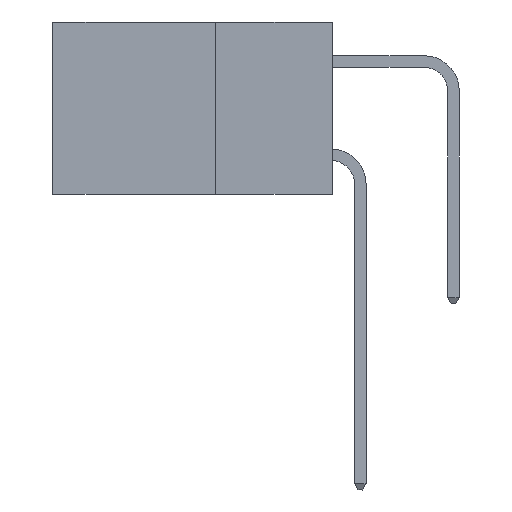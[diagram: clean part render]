
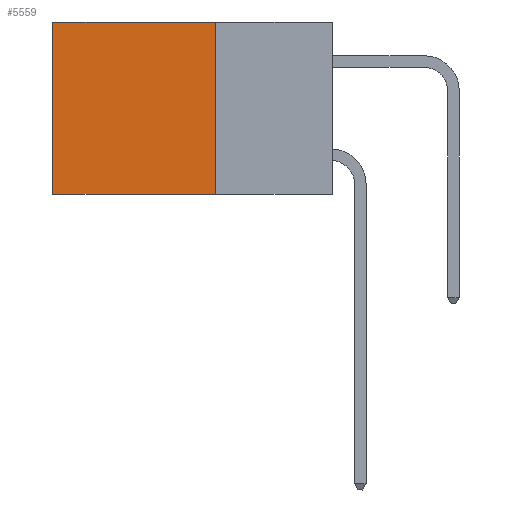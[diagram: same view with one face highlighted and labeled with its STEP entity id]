
A CAD part, left-side view. The second image highlights one B-rep face of the part: STEP entity #5559.
In plain terms, the highlighted planar face has unit normal (-1, 0, 0).
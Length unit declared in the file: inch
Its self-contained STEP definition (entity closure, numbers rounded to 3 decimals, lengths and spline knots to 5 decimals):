
#64 = VECTOR ( 'NONE', #7704, 39.37008 ) ;
#739 = EDGE_CURVE ( 'NONE', #13277, #2983, #9122, .T. ) ;
#1317 = ORIENTED_EDGE ( 'NONE', *, *, #3374, .F. ) ;
#1428 = LINE ( 'NONE', #6921, #12883 ) ;
#2800 = ORIENTED_EDGE ( 'NONE', *, *, #9118, .F. ) ;
#2983 = VERTEX_POINT ( 'NONE', #4176 ) ;
#3374 = EDGE_CURVE ( 'NONE', #14241, #4926, #1428, .T. ) ;
#3764 = DIRECTION ( 'NONE',  ( 0., 1., 0. ) ) ;
#4176 = CARTESIAN_POINT ( 'NONE',  ( 0.298, 0.6, -0.37 ) ) ;
#4782 = EDGE_CURVE ( 'NONE', #14241, #13277, #8003, .T. ) ;
#4926 = VERTEX_POINT ( 'NONE', #6750 ) ;
#4992 = VECTOR ( 'NONE', #11060, 39.37008 ) ;
#5083 = EDGE_LOOP ( 'NONE', ( #9729, #2800, #1317, #12894 ) ) ;
#5559 = ADVANCED_FACE ( 'NONE', ( #12817 ), #8153, .F. ) ;
#5856 = DIRECTION ( 'NONE',  ( 0., 0., -1. ) ) ;
#6750 = CARTESIAN_POINT ( 'NONE',  ( 0.298, 0.25, -0.37 ) ) ;
#6921 = CARTESIAN_POINT ( 'NONE',  ( 0.298, 0.25, 0. ) ) ;
#7004 = CARTESIAN_POINT ( 'NONE',  ( 0.298, 0.6, 0. ) ) ;
#7439 = CARTESIAN_POINT ( 'NONE',  ( 0.298, 0.25, 0. ) ) ;
#7616 = AXIS2_PLACEMENT_3D ( 'NONE', #8062, #13760, #13737 ) ;
#7653 = VECTOR ( 'NONE', #3764, 39.37008 ) ;
#7704 = DIRECTION ( 'NONE',  ( 0., 0., -1. ) ) ;
#8003 = LINE ( 'NONE', #7439, #7653 ) ;
#8062 = CARTESIAN_POINT ( 'NONE',  ( 0.298, 0.25, 0. ) ) ;
#8153 = PLANE ( 'NONE',  #7616 ) ;
#9118 = EDGE_CURVE ( 'NONE', #4926, #2983, #10864, .T. ) ;
#9122 = LINE ( 'NONE', #11102, #64 ) ;
#9729 = ORIENTED_EDGE ( 'NONE', *, *, #739, .T. ) ;
#9960 = CARTESIAN_POINT ( 'NONE',  ( 0.298, 0.25, -0.37 ) ) ;
#10864 = LINE ( 'NONE', #9960, #4992 ) ;
#11060 = DIRECTION ( 'NONE',  ( 0., 1., 0. ) ) ;
#11102 = CARTESIAN_POINT ( 'NONE',  ( 0.298, 0.6, 0. ) ) ;
#12817 = FACE_OUTER_BOUND ( 'NONE', #5083, .T. ) ;
#12883 = VECTOR ( 'NONE', #5856, 39.37008 ) ;
#12894 = ORIENTED_EDGE ( 'NONE', *, *, #4782, .T. ) ;
#13277 = VERTEX_POINT ( 'NONE', #7004 ) ;
#13737 = DIRECTION ( 'NONE',  ( 0., 0., -1. ) ) ;
#13760 = DIRECTION ( 'NONE',  ( 1., 0., 0. ) ) ;
#13920 = CARTESIAN_POINT ( 'NONE',  ( 0.298, 0.25, 0. ) ) ;
#14241 = VERTEX_POINT ( 'NONE', #13920 ) ;
